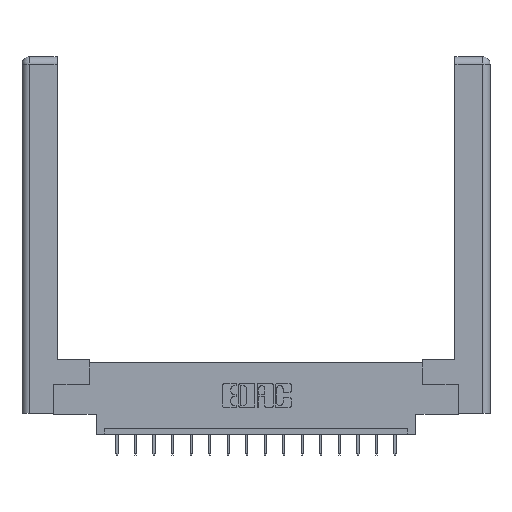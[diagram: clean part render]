
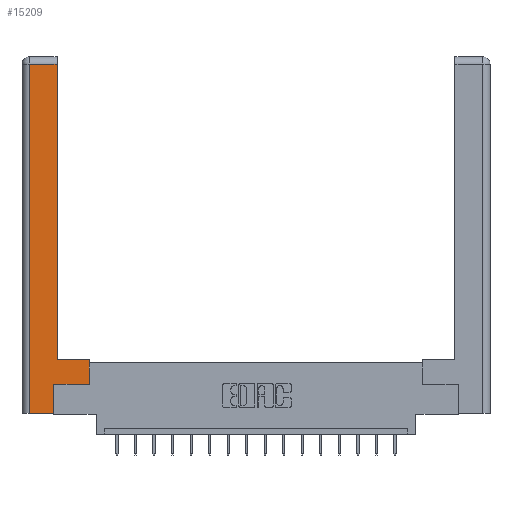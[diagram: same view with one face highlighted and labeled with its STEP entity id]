
A CAD part, top view. The second image highlights one B-rep face of the part: STEP entity #15209.
In plain terms, the highlighted planar face has unit normal (0, 0, 1).
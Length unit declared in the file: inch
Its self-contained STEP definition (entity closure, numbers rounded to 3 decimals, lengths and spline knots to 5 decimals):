
#203 = LINE ( 'NONE', #2363, #16593 ) ;
#224 = DIRECTION ( 'NONE',  ( 0., 1., 0. ) ) ;
#652 = ORIENTED_EDGE ( 'NONE', *, *, #4624, .T. ) ;
#909 = LINE ( 'NONE', #4500, #10952 ) ;
#1255 = VERTEX_POINT ( 'NONE', #14373 ) ;
#1642 = EDGE_CURVE ( 'NONE', #14582, #10195, #11832, .T. ) ;
#2125 = EDGE_LOOP ( 'NONE', ( #6309, #11917, #652, #9365, #10192, #11640, #13502, #15041 ) ) ;
#2337 = EDGE_CURVE ( 'NONE', #1255, #6698, #909, .T. ) ;
#2363 = CARTESIAN_POINT ( 'NONE',  ( 0.565, 0.45, 0. ) ) ;
#3217 = LINE ( 'NONE', #12840, #9288 ) ;
#3246 = VERTEX_POINT ( 'NONE', #17435 ) ;
#3994 = VECTOR ( 'NONE', #4382, 39.37008 ) ;
#4382 = DIRECTION ( 'NONE',  ( 1., 0., 0. ) ) ;
#4500 = CARTESIAN_POINT ( 'NONE',  ( 0.295, 3., 0. ) ) ;
#4624 = EDGE_CURVE ( 'NONE', #13738, #3246, #4709, .T. ) ;
#4709 = LINE ( 'NONE', #7623, #12355 ) ;
#5394 = DIRECTION ( 'NONE',  ( 0., 0., -1. ) ) ;
#5981 = VECTOR ( 'NONE', #15667, 39.37008 ) ;
#6309 = ORIENTED_EDGE ( 'NONE', *, *, #2337, .T. ) ;
#6698 = VERTEX_POINT ( 'NONE', #13768 ) ;
#6705 = PLANE ( 'NONE',  #11913 ) ;
#7321 = CARTESIAN_POINT ( 'NONE',  ( 0.0615, 2.94, 0. ) ) ;
#7585 = VERTEX_POINT ( 'NONE', #15258 ) ;
#7614 = DIRECTION ( 'NONE',  ( 0., 1., 0. ) ) ;
#7623 = CARTESIAN_POINT ( 'NONE',  ( 0.0615, 0., 0. ) ) ;
#7815 = CARTESIAN_POINT ( 'NONE',  ( 0.0615, 2.94, 0. ) ) ;
#8517 = EDGE_CURVE ( 'NONE', #10195, #7585, #203, .T. ) ;
#8951 = LINE ( 'NONE', #7321, #10951 ) ;
#9288 = VECTOR ( 'NONE', #12777, 39.37008 ) ;
#9365 = ORIENTED_EDGE ( 'NONE', *, *, #12417, .T. ) ;
#9699 = EDGE_CURVE ( 'NONE', #7585, #1255, #10771, .T. ) ;
#10192 = ORIENTED_EDGE ( 'NONE', *, *, #14087, .T. ) ;
#10195 = VERTEX_POINT ( 'NONE', #11626 ) ;
#10478 = LINE ( 'NONE', #14290, #14238 ) ;
#10528 = CARTESIAN_POINT ( 'NONE',  ( 0.265, 0.245, 0. ) ) ;
#10771 = LINE ( 'NONE', #12831, #5981 ) ;
#10951 = VECTOR ( 'NONE', #17184, 39.37008 ) ;
#10952 = VECTOR ( 'NONE', #224, 39.37008 ) ;
#11424 = CARTESIAN_POINT ( 'NONE',  ( 0.565, 0.245, 0. ) ) ;
#11626 = CARTESIAN_POINT ( 'NONE',  ( 0.565, 0.245, 0. ) ) ;
#11640 = ORIENTED_EDGE ( 'NONE', *, *, #1642, .T. ) ;
#11832 = LINE ( 'NONE', #11424, #3994 ) ;
#11913 = AXIS2_PLACEMENT_3D ( 'NONE', #13762, #5394, #15175 ) ;
#11917 = ORIENTED_EDGE ( 'NONE', *, *, #16008, .T. ) ;
#12255 = CARTESIAN_POINT ( 'NONE',  ( 0.265, 0., 0. ) ) ;
#12355 = VECTOR ( 'NONE', #13473, 39.37008 ) ;
#12417 = EDGE_CURVE ( 'NONE', #3246, #17469, #10478, .T. ) ;
#12777 = DIRECTION ( 'NONE',  ( 0., 1., 0. ) ) ;
#12831 = CARTESIAN_POINT ( 'NONE',  ( 0.295, 0.45, 0. ) ) ;
#12840 = CARTESIAN_POINT ( 'NONE',  ( 0.265, 0.245, 0. ) ) ;
#13473 = DIRECTION ( 'NONE',  ( 0., -1., 0. ) ) ;
#13502 = ORIENTED_EDGE ( 'NONE', *, *, #8517, .T. ) ;
#13738 = VERTEX_POINT ( 'NONE', #7815 ) ;
#13762 = CARTESIAN_POINT ( 'NONE',  ( 0., 0., 0. ) ) ;
#13768 = CARTESIAN_POINT ( 'NONE',  ( 0.295, 2.94, 0. ) ) ;
#14087 = EDGE_CURVE ( 'NONE', #17469, #14582, #3217, .T. ) ;
#14238 = VECTOR ( 'NONE', #15441, 39.37008 ) ;
#14290 = CARTESIAN_POINT ( 'NONE',  ( 0.265, 0., 0. ) ) ;
#14373 = CARTESIAN_POINT ( 'NONE',  ( 0.295, 0.45, 0. ) ) ;
#14582 = VERTEX_POINT ( 'NONE', #10528 ) ;
#15041 = ORIENTED_EDGE ( 'NONE', *, *, #9699, .T. ) ;
#15175 = DIRECTION ( 'NONE',  ( -1., 0., 0. ) ) ;
#15209 = ADVANCED_FACE ( 'NONE', ( #16894 ), #6705, .F. ) ;
#15258 = CARTESIAN_POINT ( 'NONE',  ( 0.565, 0.45, 0. ) ) ;
#15441 = DIRECTION ( 'NONE',  ( 1., 0., 0. ) ) ;
#15667 = DIRECTION ( 'NONE',  ( -1., 0., 0. ) ) ;
#16008 = EDGE_CURVE ( 'NONE', #6698, #13738, #8951, .T. ) ;
#16593 = VECTOR ( 'NONE', #7614, 39.37008 ) ;
#16894 = FACE_OUTER_BOUND ( 'NONE', #2125, .T. ) ;
#17184 = DIRECTION ( 'NONE',  ( -1., 0., 0. ) ) ;
#17435 = CARTESIAN_POINT ( 'NONE',  ( 0.0615, 0., 0. ) ) ;
#17469 = VERTEX_POINT ( 'NONE', #12255 ) ;
